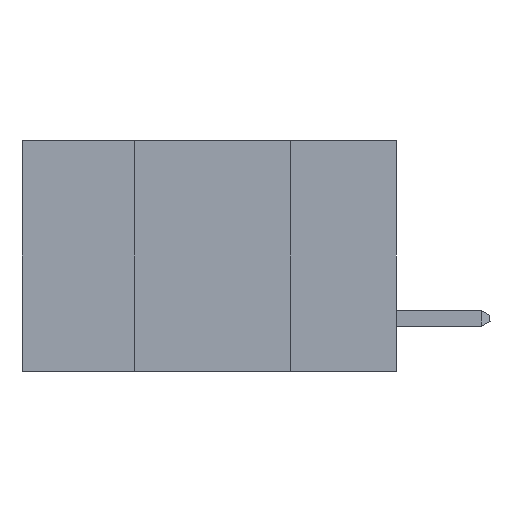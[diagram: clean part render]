
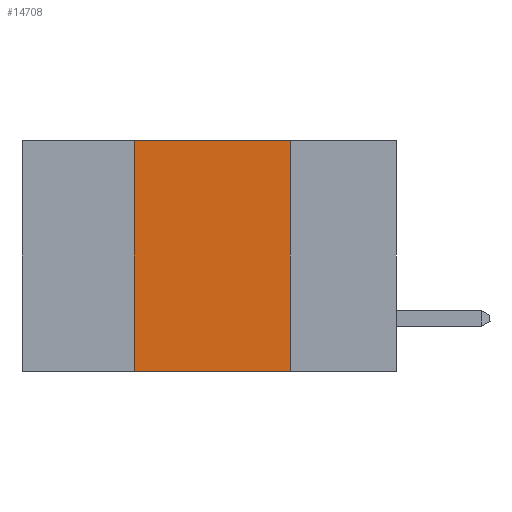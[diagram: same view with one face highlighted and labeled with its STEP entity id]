
A CAD part, left-side view. The second image highlights one B-rep face of the part: STEP entity #14708.
In plain terms, the highlighted planar face has unit normal (-1, 0, 0).
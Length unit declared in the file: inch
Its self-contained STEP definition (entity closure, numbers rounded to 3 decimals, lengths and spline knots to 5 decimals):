
#1118 = LINE ( 'NONE', #23181, #13165 ) ;
#1214 = CARTESIAN_POINT ( 'NONE',  ( 0., 0.42, 0. ) ) ;
#1682 = FACE_OUTER_BOUND ( 'NONE', #12360, .T. ) ;
#2836 = CARTESIAN_POINT ( 'NONE',  ( 0., 0.6, 0. ) ) ;
#3988 = VECTOR ( 'NONE', #16598, 39.37008 ) ;
#4047 = DIRECTION ( 'NONE',  ( 0., -1., 0. ) ) ;
#4273 = ORIENTED_EDGE ( 'NONE', *, *, #6055, .F. ) ;
#5247 = DIRECTION ( 'NONE',  ( 0., 0., -1. ) ) ;
#5303 = CARTESIAN_POINT ( 'NONE',  ( 0., 0.42, -0.37 ) ) ;
#5468 = CARTESIAN_POINT ( 'NONE',  ( 0., 0.6, -0.37 ) ) ;
#5696 = VECTOR ( 'NONE', #12741, 39.37008 ) ;
#6055 = EDGE_CURVE ( 'NONE', #17910, #18732, #1118, .T. ) ;
#9147 = CARTESIAN_POINT ( 'NONE',  ( 0., 0.17, 0. ) ) ;
#9495 = ORIENTED_EDGE ( 'NONE', *, *, #28935, .F. ) ;
#10170 = CARTESIAN_POINT ( 'NONE',  ( 0., 0.17, -0.37 ) ) ;
#12360 = EDGE_LOOP ( 'NONE', ( #27070, #4273, #9495, #24584 ) ) ;
#12741 = DIRECTION ( 'NONE',  ( 0., -1., 0. ) ) ;
#13165 = VECTOR ( 'NONE', #4047, 39.37008 ) ;
#14212 = AXIS2_PLACEMENT_3D ( 'NONE', #2836, #19640, #5247 ) ;
#14708 = ADVANCED_FACE ( 'NONE', ( #1682 ), #28884, .F. ) ;
#16598 = DIRECTION ( 'NONE',  ( 0., 0., -1. ) ) ;
#17910 = VERTEX_POINT ( 'NONE', #1214 ) ;
#18414 = EDGE_CURVE ( 'NONE', #22722, #29840, #24751, .T. ) ;
#18732 = VERTEX_POINT ( 'NONE', #9147 ) ;
#19640 = DIRECTION ( 'NONE',  ( 1., 0., 0. ) ) ;
#20833 = VECTOR ( 'NONE', #21107, 39.37008 ) ;
#21107 = DIRECTION ( 'NONE',  ( 0., 0., 1. ) ) ;
#21559 = LINE ( 'NONE', #30334, #20833 ) ;
#22722 = VERTEX_POINT ( 'NONE', #5303 ) ;
#23181 = CARTESIAN_POINT ( 'NONE',  ( 0., 0.6, 0. ) ) ;
#24584 = ORIENTED_EDGE ( 'NONE', *, *, #18414, .T. ) ;
#24751 = LINE ( 'NONE', #5468, #5696 ) ;
#27070 = ORIENTED_EDGE ( 'NONE', *, *, #27406, .F. ) ;
#27406 = EDGE_CURVE ( 'NONE', #18732, #29840, #29224, .T. ) ;
#28262 = CARTESIAN_POINT ( 'NONE',  ( 0., 0.17, 0. ) ) ;
#28884 = PLANE ( 'NONE',  #14212 ) ;
#28935 = EDGE_CURVE ( 'NONE', #22722, #17910, #21559, .T. ) ;
#29224 = LINE ( 'NONE', #28262, #3988 ) ;
#29840 = VERTEX_POINT ( 'NONE', #10170 ) ;
#30334 = CARTESIAN_POINT ( 'NONE',  ( 0., 0.42, 0. ) ) ;
